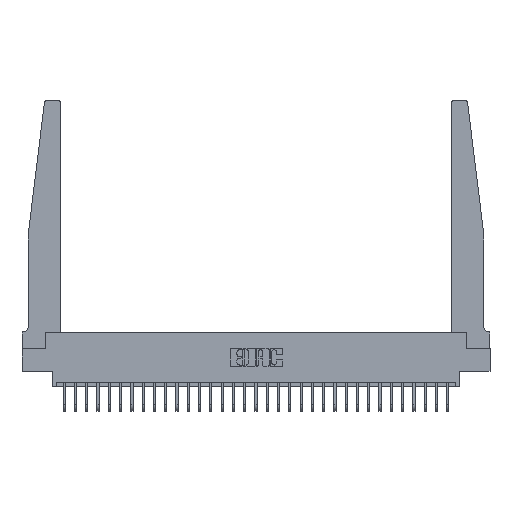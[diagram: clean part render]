
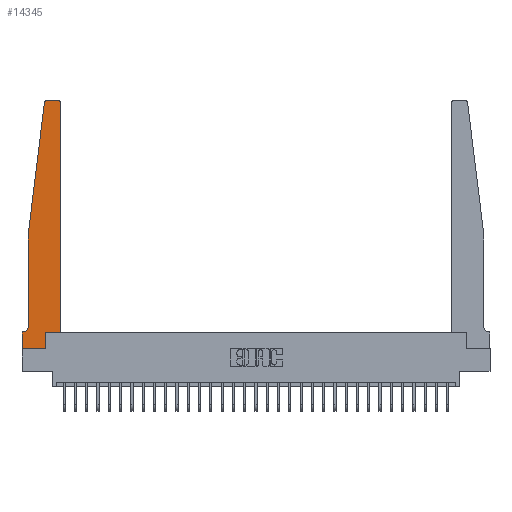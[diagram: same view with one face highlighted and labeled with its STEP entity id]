
A CAD part, top view. The second image highlights one B-rep face of the part: STEP entity #14345.
In plain terms, the highlighted planar face has unit normal (0, 0, 1).
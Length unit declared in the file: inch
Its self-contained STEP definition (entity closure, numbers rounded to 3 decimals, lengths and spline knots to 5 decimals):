
#539 = CARTESIAN_POINT ( 'NONE',  ( 0.425, 0.18, 0.37 ) ) ;
#792 = EDGE_CURVE ( 'NONE', #4622, #23571, #2683, .T. ) ;
#1201 = EDGE_CURVE ( 'NONE', #4808, #8617, #7065, .T. ) ;
#1275 = VERTEX_POINT ( 'NONE', #4434 ) ;
#2683 = LINE ( 'NONE', #18616, #16319 ) ;
#2694 = CARTESIAN_POINT ( 'NONE',  ( 0.27653, 2.75, 0.37 ) ) ;
#3196 = VECTOR ( 'NONE', #23112, 39.37008 ) ;
#3307 = CARTESIAN_POINT ( 'NONE',  ( 0.395, 2.72, 0.37 ) ) ;
#3874 = ORIENTED_EDGE ( 'NONE', *, *, #1201, .T. ) ;
#4080 = EDGE_CURVE ( 'NONE', #6505, #23133, #26489, .T. ) ;
#4086 = PLANE ( 'NONE',  #27676 ) ;
#4434 = CARTESIAN_POINT ( 'NONE',  ( 0.015, 0.1875, 0.37 ) ) ;
#4446 = CARTESIAN_POINT ( 'NONE',  ( 0., 0., 0.37 ) ) ;
#4476 = CARTESIAN_POINT ( 'NONE',  ( 0.2605, 0., 0.37 ) ) ;
#4507 = EDGE_CURVE ( 'NONE', #17643, #4622, #26829, .T. ) ;
#4622 = VERTEX_POINT ( 'NONE', #20293 ) ;
#4625 = EDGE_CURVE ( 'NONE', #24161, #24745, #10579, .T. ) ;
#4808 = VERTEX_POINT ( 'NONE', #6893 ) ;
#4871 = CARTESIAN_POINT ( 'NONE',  ( 0.065, 0.1875, 0.37 ) ) ;
#5108 = VECTOR ( 'NONE', #5750, 39.37008 ) ;
#5171 = ORIENTED_EDGE ( 'NONE', *, *, #792, .T. ) ;
#5750 = DIRECTION ( 'NONE',  ( 0., -1., 0. ) ) ;
#5778 = VECTOR ( 'NONE', #8028, 39.37008 ) ;
#5795 = LINE ( 'NONE', #9455, #21702 ) ;
#6149 = VECTOR ( 'NONE', #20321, 39.37008 ) ;
#6505 = VERTEX_POINT ( 'NONE', #12180 ) ;
#6837 = EDGE_CURVE ( 'NONE', #23571, #21150, #5795, .T. ) ;
#6893 = CARTESIAN_POINT ( 'NONE',  ( 0.425, 2.72, 0.37 ) ) ;
#7065 = CIRCLE ( 'NONE', #11742, 0.03 ) ;
#7411 = CARTESIAN_POINT ( 'NONE',  ( 0.425, 0.18, 0.37 ) ) ;
#7442 = VECTOR ( 'NONE', #17089, 39.37008 ) ;
#8028 = DIRECTION ( 'NONE',  ( -1., 0., 0. ) ) ;
#8151 = VECTOR ( 'NONE', #17450, 39.37008 ) ;
#8340 = CARTESIAN_POINT ( 'NONE',  ( 0., 0., 0.37 ) ) ;
#8557 = CARTESIAN_POINT ( 'NONE',  ( 0.27653, 2.72, 0.37 ) ) ;
#8617 = VERTEX_POINT ( 'NONE', #19436 ) ;
#9382 = ORIENTED_EDGE ( 'NONE', *, *, #15394, .T. ) ;
#9455 = CARTESIAN_POINT ( 'NONE',  ( 0.065, 1.25, 0.37 ) ) ;
#9500 = AXIS2_PLACEMENT_3D ( 'NONE', #8557, #10875, #25088 ) ;
#9856 = VECTOR ( 'NONE', #26850, 39.37008 ) ;
#9861 = ORIENTED_EDGE ( 'NONE', *, *, #21818, .T. ) ;
#10452 = CARTESIAN_POINT ( 'NONE',  ( 0.2605, 0.18, 0.37 ) ) ;
#10579 = LINE ( 'NONE', #7411, #6149 ) ;
#10765 = LINE ( 'NONE', #4871, #8151 ) ;
#10875 = DIRECTION ( 'NONE',  ( 0., 0., 1. ) ) ;
#10920 = EDGE_CURVE ( 'NONE', #24745, #4808, #11904, .T. ) ;
#11742 = AXIS2_PLACEMENT_3D ( 'NONE', #3307, #24594, #22056 ) ;
#11904 = LINE ( 'NONE', #539, #7442 ) ;
#12127 = CARTESIAN_POINT ( 'NONE',  ( 0.065, 0.2375, 0.37 ) ) ;
#12180 = CARTESIAN_POINT ( 'NONE',  ( 0., 0.1875, 0.37 ) ) ;
#12333 = ORIENTED_EDGE ( 'NONE', *, *, #4080, .T. ) ;
#14110 = ORIENTED_EDGE ( 'NONE', *, *, #24847, .T. ) ;
#14345 = ADVANCED_FACE ( 'NONE', ( #25822 ), #4086, .T. ) ;
#15394 = EDGE_CURVE ( 'NONE', #8617, #17643, #16898, .T. ) ;
#15835 = DIRECTION ( 'NONE',  ( 0., 0., 1. ) ) ;
#16319 = VECTOR ( 'NONE', #18723, 39.37008 ) ;
#16453 = ORIENTED_EDGE ( 'NONE', *, *, #29030, .T. ) ;
#16898 = LINE ( 'NONE', #17875, #5778 ) ;
#17089 = DIRECTION ( 'NONE',  ( 0., 1., 0. ) ) ;
#17383 = CARTESIAN_POINT ( 'NONE',  ( 0., 0., 0.37 ) ) ;
#17450 = DIRECTION ( 'NONE',  ( -1., 0., 0. ) ) ;
#17643 = VERTEX_POINT ( 'NONE', #2694 ) ;
#17875 = CARTESIAN_POINT ( 'NONE',  ( 0.25, 2.75, 0.37 ) ) ;
#18197 = DIRECTION ( 'NONE',  ( 1., 0., 0. ) ) ;
#18616 = CARTESIAN_POINT ( 'NONE',  ( 0.065, 1.25, 0.37 ) ) ;
#18723 = DIRECTION ( 'NONE',  ( -0.122, -0.992, 0. ) ) ;
#18920 = CARTESIAN_POINT ( 'NONE',  ( 0.015, 0.2375, 0.37 ) ) ;
#19436 = CARTESIAN_POINT ( 'NONE',  ( 0.395, 2.75, 0.37 ) ) ;
#20165 = CIRCLE ( 'NONE', #20645, 0.05 ) ;
#20293 = CARTESIAN_POINT ( 'NONE',  ( 0.24675, 2.72367, 0.37 ) ) ;
#20321 = DIRECTION ( 'NONE',  ( 1., 0., 0. ) ) ;
#20645 = AXIS2_PLACEMENT_3D ( 'NONE', #18920, #23867, #28169 ) ;
#20754 = CARTESIAN_POINT ( 'NONE',  ( 0.065, 1.25, 0.37 ) ) ;
#20878 = LINE ( 'NONE', #4446, #3196 ) ;
#20927 = CARTESIAN_POINT ( 'NONE',  ( 0.2605, 0.18, 0.37 ) ) ;
#21150 = VERTEX_POINT ( 'NONE', #12127 ) ;
#21614 = VERTEX_POINT ( 'NONE', #4476 ) ;
#21702 = VECTOR ( 'NONE', #25961, 39.37008 ) ;
#21818 = EDGE_CURVE ( 'NONE', #1275, #6505, #10765, .T. ) ;
#22056 = DIRECTION ( 'NONE',  ( 1., 0., 0. ) ) ;
#22103 = ORIENTED_EDGE ( 'NONE', *, *, #4507, .T. ) ;
#22756 = ORIENTED_EDGE ( 'NONE', *, *, #28217, .T. ) ;
#22770 = ORIENTED_EDGE ( 'NONE', *, *, #4625, .T. ) ;
#23112 = DIRECTION ( 'NONE',  ( 1., 0., 0. ) ) ;
#23133 = VERTEX_POINT ( 'NONE', #17383 ) ;
#23482 = ORIENTED_EDGE ( 'NONE', *, *, #10920, .T. ) ;
#23571 = VERTEX_POINT ( 'NONE', #20754 ) ;
#23867 = DIRECTION ( 'NONE',  ( 0., 0., -1. ) ) ;
#24161 = VERTEX_POINT ( 'NONE', #20927 ) ;
#24594 = DIRECTION ( 'NONE',  ( 0., 0., 1. ) ) ;
#24745 = VERTEX_POINT ( 'NONE', #27692 ) ;
#24847 = EDGE_CURVE ( 'NONE', #21150, #1275, #20165, .T. ) ;
#25088 = DIRECTION ( 'NONE',  ( 1., 0., 0. ) ) ;
#25822 = FACE_OUTER_BOUND ( 'NONE', #30242, .T. ) ;
#25961 = DIRECTION ( 'NONE',  ( 0., -1., 0. ) ) ;
#26489 = LINE ( 'NONE', #8340, #5108 ) ;
#26829 = CIRCLE ( 'NONE', #9500, 0.03 ) ;
#26850 = DIRECTION ( 'NONE',  ( 0., 1., 0. ) ) ;
#27676 = AXIS2_PLACEMENT_3D ( 'NONE', #29897, #15835, #18197 ) ;
#27692 = CARTESIAN_POINT ( 'NONE',  ( 0.425, 0.18, 0.37 ) ) ;
#28169 = DIRECTION ( 'NONE',  ( -1., 0., 0. ) ) ;
#28217 = EDGE_CURVE ( 'NONE', #21614, #24161, #28648, .T. ) ;
#28648 = LINE ( 'NONE', #10452, #9856 ) ;
#28888 = ORIENTED_EDGE ( 'NONE', *, *, #6837, .T. ) ;
#29030 = EDGE_CURVE ( 'NONE', #23133, #21614, #20878, .T. ) ;
#29897 = CARTESIAN_POINT ( 'NONE',  ( 0., 0.1875, 0.37 ) ) ;
#30242 = EDGE_LOOP ( 'NONE', ( #9382, #22103, #5171, #28888, #14110, #9861, #12333, #16453, #22756, #22770, #23482, #3874 ) ) ;
